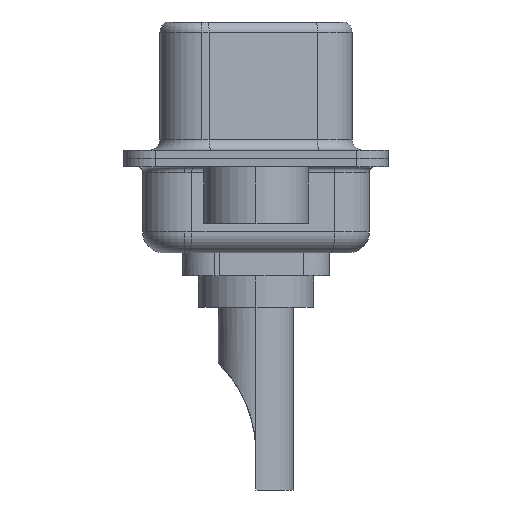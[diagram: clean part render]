
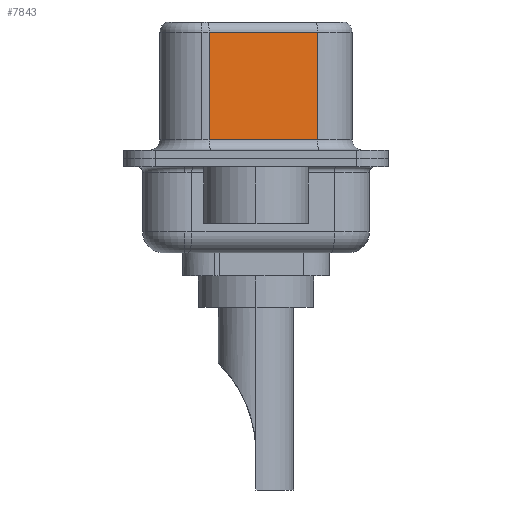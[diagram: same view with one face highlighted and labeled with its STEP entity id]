
A CAD part, left-side view. The second image highlights one B-rep face of the part: STEP entity #7843.
In plain terms, the highlighted planar face has unit normal (-0.985, -0.174, 0).
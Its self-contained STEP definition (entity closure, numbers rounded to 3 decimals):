
#478 = CARTESIAN_POINT ( 'NONE',  ( 4.565, -2.927, 6.02 ) ) ;
#861 = VECTOR ( 'NONE', #8346, 1000. ) ;
#1519 = DIRECTION ( 'NONE',  ( -0.174, 0.985, 0. ) ) ;
#1654 = EDGE_LOOP ( 'NONE', ( #15352, #11224, #11272, #10163 ) ) ;
#2963 = LINE ( 'NONE', #478, #5866 ) ;
#3302 = DIRECTION ( 'NONE',  ( 0., 0., -1. ) ) ;
#4252 = VERTEX_POINT ( 'NONE', #14729 ) ;
#4437 = CARTESIAN_POINT ( 'NONE',  ( 4.565, -2.927, 0.9 ) ) ;
#4518 = CARTESIAN_POINT ( 'NONE',  ( 3.655, 2.233, 0.9 ) ) ;
#5866 = VECTOR ( 'NONE', #10600, 1000. ) ;
#6004 = LINE ( 'NONE', #10708, #9037 ) ;
#6336 = PLANE ( 'NONE',  #7018 ) ;
#7018 = AXIS2_PLACEMENT_3D ( 'NONE', #12656, #9000, #1519 ) ;
#7843 = ADVANCED_FACE ( 'NONE', ( #15999 ), #6336, .F. ) ;
#8100 = EDGE_CURVE ( 'NONE', #4252, #8523, #8489, .T. ) ;
#8346 = DIRECTION ( 'NONE',  ( 0.174, -0.985, 0. ) ) ;
#8434 = EDGE_CURVE ( 'NONE', #9927, #4252, #2963, .T. ) ;
#8489 = LINE ( 'NONE', #10876, #12182 ) ;
#8523 = VERTEX_POINT ( 'NONE', #4518 ) ;
#9000 = DIRECTION ( 'NONE',  ( 0.985, 0.174, 0. ) ) ;
#9037 = VECTOR ( 'NONE', #11900, 1000. ) ;
#9927 = VERTEX_POINT ( 'NONE', #10211 ) ;
#10163 = ORIENTED_EDGE ( 'NONE', *, *, #14587, .T. ) ;
#10211 = CARTESIAN_POINT ( 'NONE',  ( 4.565, -2.927, 6.02 ) ) ;
#10600 = DIRECTION ( 'NONE',  ( -0.174, 0.985, 0. ) ) ;
#10708 = CARTESIAN_POINT ( 'NONE',  ( 4.565, -2.927, 6.52 ) ) ;
#10819 = LINE ( 'NONE', #13353, #861 ) ;
#10876 = CARTESIAN_POINT ( 'NONE',  ( 3.655, 2.233, 6.52 ) ) ;
#11224 = ORIENTED_EDGE ( 'NONE', *, *, #8434, .T. ) ;
#11272 = ORIENTED_EDGE ( 'NONE', *, *, #8100, .T. ) ;
#11900 = DIRECTION ( 'NONE',  ( 0., 0., -1. ) ) ;
#12182 = VECTOR ( 'NONE', #3302, 1000. ) ;
#12656 = CARTESIAN_POINT ( 'NONE',  ( 4.565, -2.927, 6.52 ) ) ;
#13353 = CARTESIAN_POINT ( 'NONE',  ( 4.565, -2.927, 0.9 ) ) ;
#13703 = VERTEX_POINT ( 'NONE', #4437 ) ;
#14434 = EDGE_CURVE ( 'NONE', #9927, #13703, #6004, .T. ) ;
#14587 = EDGE_CURVE ( 'NONE', #8523, #13703, #10819, .T. ) ;
#14729 = CARTESIAN_POINT ( 'NONE',  ( 3.655, 2.233, 6.02 ) ) ;
#15352 = ORIENTED_EDGE ( 'NONE', *, *, #14434, .F. ) ;
#15999 = FACE_OUTER_BOUND ( 'NONE', #1654, .T. ) ;
